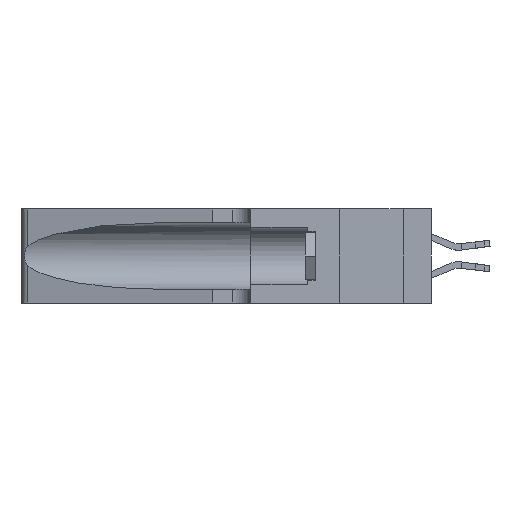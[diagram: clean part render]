
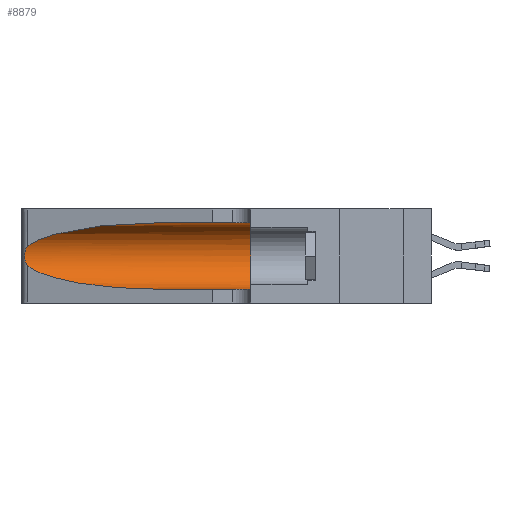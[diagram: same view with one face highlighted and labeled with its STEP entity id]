
A CAD part, left-side view. The second image highlights one B-rep face of the part: STEP entity #8879.
In plain terms, the highlighted cylindrical face has radius 3.308 mm (diameter 6.617 mm), a partial arc.
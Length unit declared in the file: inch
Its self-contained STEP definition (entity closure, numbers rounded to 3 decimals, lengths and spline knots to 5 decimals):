
#520 = CIRCLE ( 'NONE', #32258, 0.13025 ) ;
#1115 = CARTESIAN_POINT ( 'NONE',  ( 0.25487, 1.22718, 0.22369 ) ) ;
#1237 = CARTESIAN_POINT ( 'NONE',  ( 0.26018, 1.23835, 0.19895 ) ) ;
#2630 = CARTESIAN_POINT ( 'NONE',  ( 0.1305, 0.72297, 0.31525 ) ) ;
#2660 = CARTESIAN_POINT ( 'NONE',  ( 0.1305, 0.72297, 0.05475 ) ) ;
#2669 = B_SPLINE_CURVE_WITH_KNOTS ( 'NONE', 3,
 ( #1115, #31921, #15201, #34736, #18016, #1237, #20804, #4075, #23623, #6879, #26445, #9707, #29231, #12506 ),
 .UNSPECIFIED., .F., .F.,
 ( 4, 2, 2, 2, 2, 2, 4 ),
 ( 0., 0.00027, 0.00053, 0.00107, 0.0016, 0.00187, 0.00214 ),
 .UNSPECIFIED. ) ;
#2751 = CARTESIAN_POINT ( 'NONE',  ( 0.25487, 1.22718, 0.22369 ) ) ;
#2996 = CARTESIAN_POINT ( 'NONE',  ( 0.1305, 0.35, 0.31525 ) ) ;
#3119 = EDGE_CURVE ( 'NONE', #26472, #15347, #520, .T. ) ;
#3707 = CARTESIAN_POINT ( 'NONE',  ( 0.1305, 0.72297, 0.05475 ) ) ;
#3918 = CARTESIAN_POINT ( 'NONE',  ( 0.25487, 1.22718, 0.14631 ) ) ;
#4075 = CARTESIAN_POINT ( 'NONE',  ( 0.26075, 1.23896, 0.178 ) ) ;
#4521 = FACE_OUTER_BOUND ( 'NONE', #24977, .T. ) ;
#6879 = CARTESIAN_POINT ( 'NONE',  ( 0.25856, 1.23593, 0.16098 ) ) ;
#8435 = ORIENTED_EDGE ( 'NONE', *, *, #3119, .F. ) ;
#8879 = ADVANCED_FACE ( 'NONE', ( #4521 ), #25083, .F. ) ;
#9707 = CARTESIAN_POINT ( 'NONE',  ( 0.25639, 1.23186, 0.15144 ) ) ;
#10017 = VERTEX_POINT ( 'NONE', #3707 ) ;
#10056 = CARTESIAN_POINT ( 'NONE',  ( 0.1305, 1.61858, 0.31525 ) ) ;
#10098 = EDGE_CURVE ( 'NONE', #12646, #18532, #2669, .T. ) ;
#10149 = DIRECTION ( 'NONE',  ( 0., -1., 0. ) ) ;
#11472 = ORIENTED_EDGE ( 'NONE', *, *, #10098, .T. ) ;
#11786 = VECTOR ( 'NONE', #28750, 39.37008 ) ;
#12506 = CARTESIAN_POINT ( 'NONE',  ( 0.25487, 1.22718, 0.14631 ) ) ;
#12646 = VERTEX_POINT ( 'NONE', #34722 ) ;
#12954 = DIRECTION ( 'NONE',  ( 0., 0., -1. ) ) ;
#14120 = ORIENTED_EDGE ( 'NONE', *, *, #33754, .T. ) ;
#15201 = CARTESIAN_POINT ( 'NONE',  ( 0.25639, 1.23184, 0.21858 ) ) ;
#15347 = VERTEX_POINT ( 'NONE', #31952 ) ;
#15671 = DIRECTION ( 'NONE',  ( 0., 1., 0. ) ) ;
#15855 = ORIENTED_EDGE ( 'NONE', *, *, #29666, .F. ) ;
#16794 =( BOUNDED_CURVE ( )  B_SPLINE_CURVE ( 3, ( #2630, #30612, #19482, #2751 ),
 .UNSPECIFIED., .F., .F. ) 
 B_SPLINE_CURVE_WITH_KNOTS ( ( 4, 4 ),
 ( 1.5708, 2.84003 ),
 .UNSPECIFIED. ) 
 CURVE ( )  GEOMETRIC_REPRESENTATION_ITEM ( )  RATIONAL_B_SPLINE_CURVE ( ( 1., 0.87, 0.87, 1. ) ) 
 REPRESENTATION_ITEM ( '' )  );
#17154 = ORIENTED_EDGE ( 'NONE', *, *, #28396, .T. ) ;
#18016 = CARTESIAN_POINT ( 'NONE',  ( 0.25854, 1.2359, 0.20912 ) ) ;
#18338 = LINE ( 'NONE', #20321, #11786 ) ;
#18532 = VERTEX_POINT ( 'NONE', #3918 ) ;
#18748 = LINE ( 'NONE', #10056, #27072 ) ;
#19388 = CARTESIAN_POINT ( 'NONE',  ( 0.18966, 0.96281, 0.05475 ) ) ;
#19482 = CARTESIAN_POINT ( 'NONE',  ( 0.2373, 1.15595, 0.28018 ) ) ;
#20321 = CARTESIAN_POINT ( 'NONE',  ( 0.1305, 1.61858, 0.05475 ) ) ;
#20588 =( BOUNDED_CURVE ( )  B_SPLINE_CURVE ( 3, ( #30515, #22091, #19388, #2660 ),
 .UNSPECIFIED., .F., .F. ) 
 B_SPLINE_CURVE_WITH_KNOTS ( ( 4, 4 ),
 ( 3.44316, 4.71239 ),
 .UNSPECIFIED. ) 
 CURVE ( )  GEOMETRIC_REPRESENTATION_ITEM ( )  RATIONAL_B_SPLINE_CURVE ( ( 1., 0.87, 0.87, 1. ) ) 
 REPRESENTATION_ITEM ( '' )  );
#20804 = CARTESIAN_POINT ( 'NONE',  ( 0.26075, 1.23896, 0.19203 ) ) ;
#21144 = VERTEX_POINT ( 'NONE', #28839 ) ;
#21523 = ORIENTED_EDGE ( 'NONE', *, *, #29461, .T. ) ;
#22091 = CARTESIAN_POINT ( 'NONE',  ( 0.2373, 1.15595, 0.08982 ) ) ;
#23623 = CARTESIAN_POINT ( 'NONE',  ( 0.26017, 1.23833, 0.17102 ) ) ;
#23986 = DIRECTION ( 'NONE',  ( 0., -1., 0. ) ) ;
#24201 = AXIS2_PLACEMENT_3D ( 'NONE', #35296, #10149, #12954 ) ;
#24977 = EDGE_LOOP ( 'NONE', ( #17154, #11472, #14120, #21523, #8435, #15855 ) ) ;
#25083 = CYLINDRICAL_SURFACE ( 'NONE', #24201, 0.13025 ) ;
#26445 = CARTESIAN_POINT ( 'NONE',  ( 0.25789, 1.23486, 0.15765 ) ) ;
#26472 = VERTEX_POINT ( 'NONE', #2996 ) ;
#27072 = VECTOR ( 'NONE', #23986, 39.37008 ) ;
#28396 = EDGE_CURVE ( 'NONE', #21144, #12646, #16794, .T. ) ;
#28750 = DIRECTION ( 'NONE',  ( 0., -1., 0. ) ) ;
#28839 = CARTESIAN_POINT ( 'NONE',  ( 0.1305, 0.72297, 0.31525 ) ) ;
#29231 = CARTESIAN_POINT ( 'NONE',  ( 0.25555, 1.22993, 0.14849 ) ) ;
#29461 = EDGE_CURVE ( 'NONE', #10017, #15347, #18338, .T. ) ;
#29666 = EDGE_CURVE ( 'NONE', #21144, #26472, #18748, .T. ) ;
#30515 = CARTESIAN_POINT ( 'NONE',  ( 0.25487, 1.22718, 0.14631 ) ) ;
#30612 = CARTESIAN_POINT ( 'NONE',  ( 0.18966, 0.96281, 0.31525 ) ) ;
#31921 = CARTESIAN_POINT ( 'NONE',  ( 0.25555, 1.22994, 0.2215 ) ) ;
#31952 = CARTESIAN_POINT ( 'NONE',  ( 0.1305, 0.35, 0.05475 ) ) ;
#32258 = AXIS2_PLACEMENT_3D ( 'NONE', #32387, #15671, #35199 ) ;
#32387 = CARTESIAN_POINT ( 'NONE',  ( 0.1305, 0.35, 0.185 ) ) ;
#33754 = EDGE_CURVE ( 'NONE', #18532, #10017, #20588, .T. ) ;
#34722 = CARTESIAN_POINT ( 'NONE',  ( 0.25487, 1.22718, 0.22369 ) ) ;
#34736 = CARTESIAN_POINT ( 'NONE',  ( 0.25787, 1.23484, 0.2124 ) ) ;
#35199 = DIRECTION ( 'NONE',  ( 0., 0., 1. ) ) ;
#35296 = CARTESIAN_POINT ( 'NONE',  ( 0.1305, 1.61858, 0.185 ) ) ;
